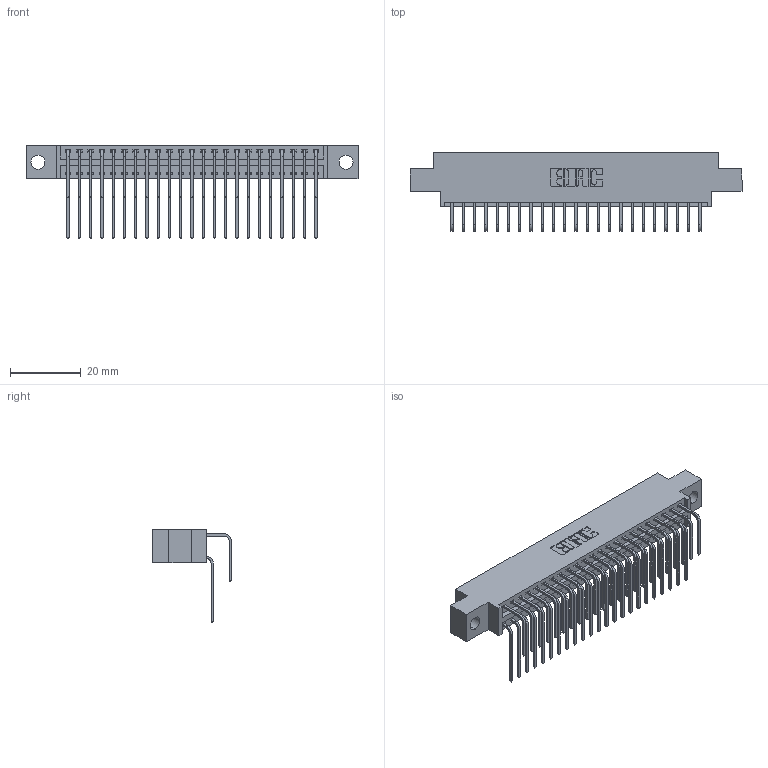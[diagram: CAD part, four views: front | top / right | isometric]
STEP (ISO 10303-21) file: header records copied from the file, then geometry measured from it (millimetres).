
FILE_DESCRIPTION (( 'STEP AP203' ), '1' );
FILE_NAME ('346-046-558-804.STEP', '2022-05-20T20:31:20', ( '' ), ( '' ), 'SwSTEP 2.0', 'SolidWorks 2020', '' );
FILE_SCHEMA (( 'CONFIG_CONTROL_DESIGN' ));
Length unit declared in the file: inch
Products named in the file (4): 345-292-001_558 Tail - 2; 346 Part_0.170 Offset - 0.156 Dia-TH; 345-292-001_558 559 Tail - 1; 346-046-558-804
Assembly tree (47 placements, depth 2):
  346-046-558-804
    346 Part_0.170 Offset - 0.156 Dia-TH
    345-292-001_558 559 Tail - 1  x23
    345-292-001_558 Tail - 2  x23
Bounding box: 93.6 x 22.16 x 26.16 mm (x, y, z)
Volume: 8984.3 mm3; surface area: 13351.4 mm2
Topology: 47 solids, 47 shells, 2624 faces, 7783 edges, 5126 vertices
Faces by surface type: plane 1796, cylinder 828
Entity records: 19903 total; most frequent: CARTESIAN_POINT 3365, ORIENTED_EDGE 3246, DIRECTION 2987, EDGE_CURVE 1623, LINE 1359, VECTOR 1359, VERTEX_POINT 1078, AXIS2_PLACEMENT_3D 814
